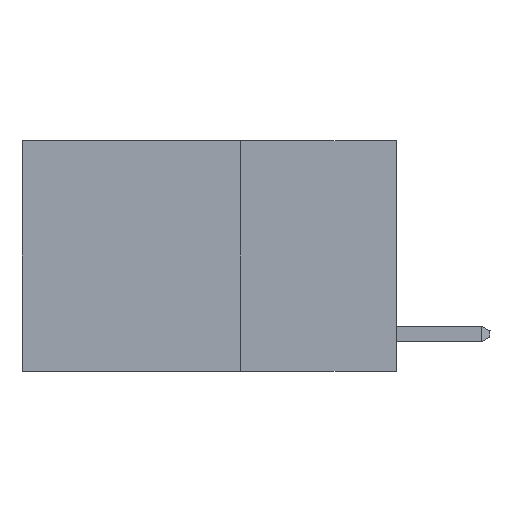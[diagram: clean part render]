
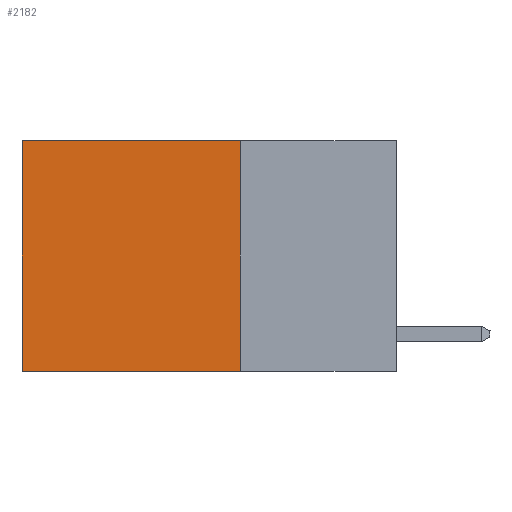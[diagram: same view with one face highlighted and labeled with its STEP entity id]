
A CAD part, left-side view. The second image highlights one B-rep face of the part: STEP entity #2182.
In plain terms, the highlighted planar face has unit normal (-1, 0, 0).
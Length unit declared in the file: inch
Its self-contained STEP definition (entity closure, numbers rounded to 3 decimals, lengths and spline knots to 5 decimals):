
#43 = EDGE_CURVE ( 'NONE', #1931, #5316, #6637, .T. ) ;
#122 = DIRECTION ( 'NONE',  ( 0., 0., -1. ) ) ;
#1105 = VECTOR ( 'NONE', #7105, 39.37008 ) ;
#1818 = EDGE_LOOP ( 'NONE', ( #4491, #4281, #10697, #12032 ) ) ;
#1931 = VERTEX_POINT ( 'NONE', #7178 ) ;
#2182 = ADVANCED_FACE ( 'NONE', ( #14050 ), #2405, .F. ) ;
#2405 = PLANE ( 'NONE',  #13988 ) ;
#3017 = VERTEX_POINT ( 'NONE', #5695 ) ;
#3071 = VECTOR ( 'NONE', #4572, 39.37008 ) ;
#3490 = CARTESIAN_POINT ( 'NONE',  ( 0.2625, 0.25, 0. ) ) ;
#4281 = ORIENTED_EDGE ( 'NONE', *, *, #10180, .F. ) ;
#4491 = ORIENTED_EDGE ( 'NONE', *, *, #43, .T. ) ;
#4537 = CARTESIAN_POINT ( 'NONE',  ( 0.2625, 0.25, 0. ) ) ;
#4565 = VERTEX_POINT ( 'NONE', #5918 ) ;
#4572 = DIRECTION ( 'NONE',  ( 0., 1., 0. ) ) ;
#4588 = DIRECTION ( 'NONE',  ( 1., 0., 0. ) ) ;
#5297 = CARTESIAN_POINT ( 'NONE',  ( 0.2625, 0.6, -0.37 ) ) ;
#5316 = VERTEX_POINT ( 'NONE', #5297 ) ;
#5509 = CARTESIAN_POINT ( 'NONE',  ( 0.2625, 0.6, 0. ) ) ;
#5695 = CARTESIAN_POINT ( 'NONE',  ( 0.2625, 0.25, 0. ) ) ;
#5918 = CARTESIAN_POINT ( 'NONE',  ( 0.2625, 0.25, -0.37 ) ) ;
#6033 = CARTESIAN_POINT ( 'NONE',  ( 0.2625, 0.25, 0. ) ) ;
#6637 = LINE ( 'NONE', #5509, #13395 ) ;
#6769 = DIRECTION ( 'NONE',  ( 0., 0., -1. ) ) ;
#7105 = DIRECTION ( 'NONE',  ( 0., 0., -1. ) ) ;
#7178 = CARTESIAN_POINT ( 'NONE',  ( 0.2625, 0.6, 0. ) ) ;
#7587 = DIRECTION ( 'NONE',  ( 0., 1., 0. ) ) ;
#7643 = EDGE_CURVE ( 'NONE', #3017, #1931, #10416, .T. ) ;
#7735 = LINE ( 'NONE', #8615, #10343 ) ;
#8615 = CARTESIAN_POINT ( 'NONE',  ( 0.2625, 0.25, -0.37 ) ) ;
#10180 = EDGE_CURVE ( 'NONE', #4565, #5316, #7735, .T. ) ;
#10343 = VECTOR ( 'NONE', #7587, 39.37008 ) ;
#10416 = LINE ( 'NONE', #3490, #3071 ) ;
#10697 = ORIENTED_EDGE ( 'NONE', *, *, #13150, .F. ) ;
#11025 = LINE ( 'NONE', #6033, #1105 ) ;
#12032 = ORIENTED_EDGE ( 'NONE', *, *, #7643, .T. ) ;
#13150 = EDGE_CURVE ( 'NONE', #3017, #4565, #11025, .T. ) ;
#13395 = VECTOR ( 'NONE', #122, 39.37008 ) ;
#13988 = AXIS2_PLACEMENT_3D ( 'NONE', #4537, #4588, #6769 ) ;
#14050 = FACE_OUTER_BOUND ( 'NONE', #1818, .T. ) ;
